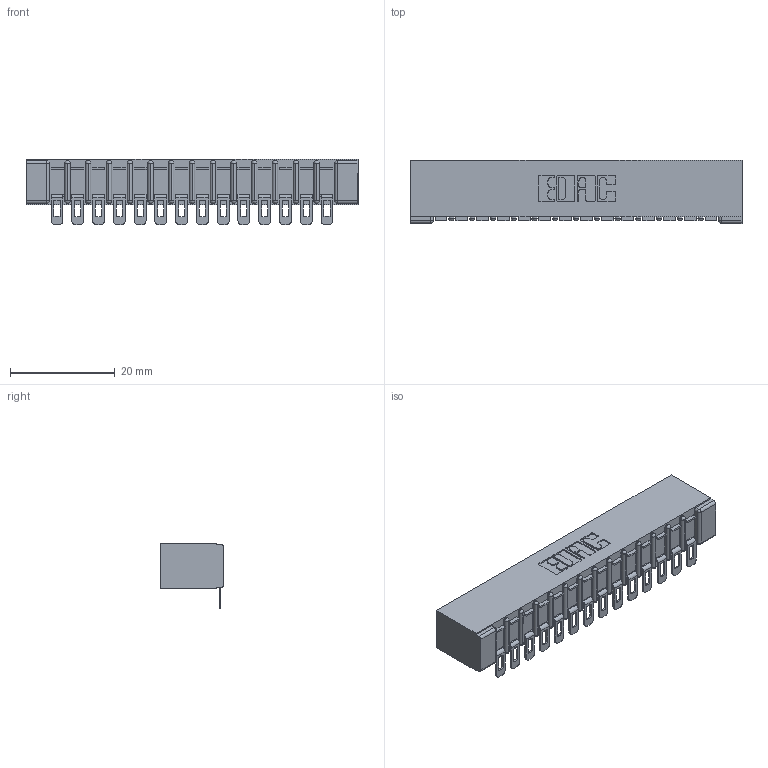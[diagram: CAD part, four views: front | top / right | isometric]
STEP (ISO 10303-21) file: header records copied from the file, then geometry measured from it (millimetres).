
FILE_DESCRIPTION (( 'STEP AP203' ), '1' );
FILE_NAME ('357-014-554-101.STEP', '2019-09-16T20:01:59', ( '' ), ( '' ), 'SwSTEP 2.0', 'SolidWorks 2016', '' );
FILE_SCHEMA (( 'CONFIG_CONTROL_DESIGN' ));
Length unit declared in the file: inch
Products named in the file (3): 307 Part_No Mounting Lugs; 357-014-554-101; 307-290-002_554
Assembly tree (15 placements, depth 2):
  357-014-554-101
    307 Part_No Mounting Lugs
    307-290-002_554  x14
Bounding box: 63.35 x 12.01 x 12.52 mm (x, y, z)
Volume: 4425.2 mm3; surface area: 8168.8 mm2
Topology: 15 solids, 15 shells, 1259 faces, 3841 edges, 2518 vertices
Faces by surface type: plane 710, cylinder 519, sphere 30
Entity records: 16141 total; most frequent: CARTESIAN_POINT 2718, ORIENTED_EDGE 2708, DIRECTION 2658, EDGE_CURVE 1354, VECTOR 1018, LINE 1018, VERTEX_POINT 880, AXIS2_PLACEMENT_3D 820
